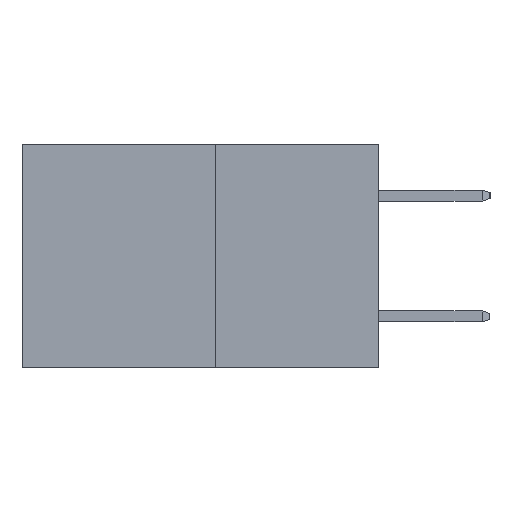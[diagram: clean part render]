
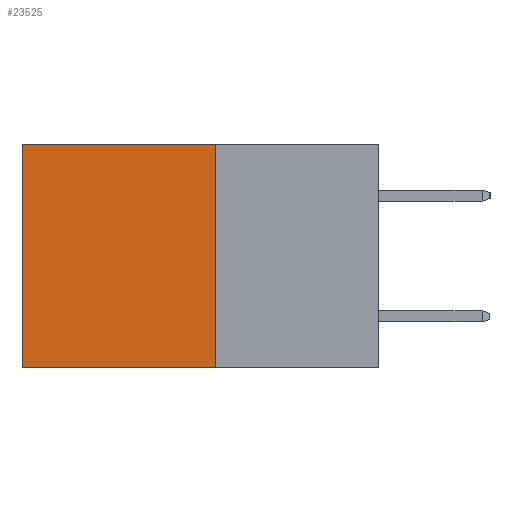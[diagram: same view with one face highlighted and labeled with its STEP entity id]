
A CAD part, left-side view. The second image highlights one B-rep face of the part: STEP entity #23525.
In plain terms, the highlighted planar face has unit normal (-1, 0, 0).
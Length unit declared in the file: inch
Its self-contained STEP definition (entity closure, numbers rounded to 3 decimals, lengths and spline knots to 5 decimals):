
#61 = CARTESIAN_POINT ( 'NONE',  ( 0.277, 0.59, -0.37 ) ) ;
#1614 = VERTEX_POINT ( 'NONE', #10186 ) ;
#1696 = LINE ( 'NONE', #5671, #20750 ) ;
#1973 = DIRECTION ( 'NONE',  ( 0., 0., -1. ) ) ;
#2645 = ORIENTED_EDGE ( 'NONE', *, *, #18615, .F. ) ;
#3099 = EDGE_CURVE ( 'NONE', #1614, #5830, #13206, .T. ) ;
#3229 = EDGE_LOOP ( 'NONE', ( #12331, #8450, #2645, #23108 ) ) ;
#4035 = VECTOR ( 'NONE', #1973, 39.37008 ) ;
#5671 = CARTESIAN_POINT ( 'NONE',  ( 0.277, 0.27, 0. ) ) ;
#5830 = VERTEX_POINT ( 'NONE', #10766 ) ;
#7392 = PLANE ( 'NONE',  #22136 ) ;
#7567 = DIRECTION ( 'NONE',  ( 0., 1., 0. ) ) ;
#8450 = ORIENTED_EDGE ( 'NONE', *, *, #3099, .F. ) ;
#9294 = DIRECTION ( 'NONE',  ( 0., 0., -1. ) ) ;
#10186 = CARTESIAN_POINT ( 'NONE',  ( 0.277, 0.27, -0.37 ) ) ;
#10620 = CARTESIAN_POINT ( 'NONE',  ( 0.277, 0.27, -0.37 ) ) ;
#10766 = CARTESIAN_POINT ( 'NONE',  ( 0.277, 0.59, -0.37 ) ) ;
#11030 = VERTEX_POINT ( 'NONE', #22374 ) ;
#12325 = DIRECTION ( 'NONE',  ( 0., 1., 0. ) ) ;
#12331 = ORIENTED_EDGE ( 'NONE', *, *, #12889, .T. ) ;
#12350 = CARTESIAN_POINT ( 'NONE',  ( 0.277, 0.27, -0.37 ) ) ;
#12525 = DIRECTION ( 'NONE',  ( 0., 0., -1. ) ) ;
#12889 = EDGE_CURVE ( 'NONE', #22250, #5830, #14140, .T. ) ;
#13206 = LINE ( 'NONE', #12350, #22714 ) ;
#14140 = LINE ( 'NONE', #61, #4035 ) ;
#14690 = VECTOR ( 'NONE', #12525, 39.37008 ) ;
#18615 = EDGE_CURVE ( 'NONE', #11030, #1614, #20359, .T. ) ;
#18989 = FACE_OUTER_BOUND ( 'NONE', #3229, .T. ) ;
#20359 = LINE ( 'NONE', #10620, #14690 ) ;
#20668 = DIRECTION ( 'NONE',  ( 1., 0., 0. ) ) ;
#20750 = VECTOR ( 'NONE', #7567, 39.37008 ) ;
#22136 = AXIS2_PLACEMENT_3D ( 'NONE', #24333, #20668, #9294 ) ;
#22250 = VERTEX_POINT ( 'NONE', #24141 ) ;
#22374 = CARTESIAN_POINT ( 'NONE',  ( 0.277, 0.27, 0. ) ) ;
#22714 = VECTOR ( 'NONE', #12325, 39.37008 ) ;
#23108 = ORIENTED_EDGE ( 'NONE', *, *, #24317, .T. ) ;
#23525 = ADVANCED_FACE ( 'NONE', ( #18989 ), #7392, .F. ) ;
#24141 = CARTESIAN_POINT ( 'NONE',  ( 0.277, 0.59, 0. ) ) ;
#24317 = EDGE_CURVE ( 'NONE', #11030, #22250, #1696, .T. ) ;
#24333 = CARTESIAN_POINT ( 'NONE',  ( 0.277, 0.27, -0.37 ) ) ;
